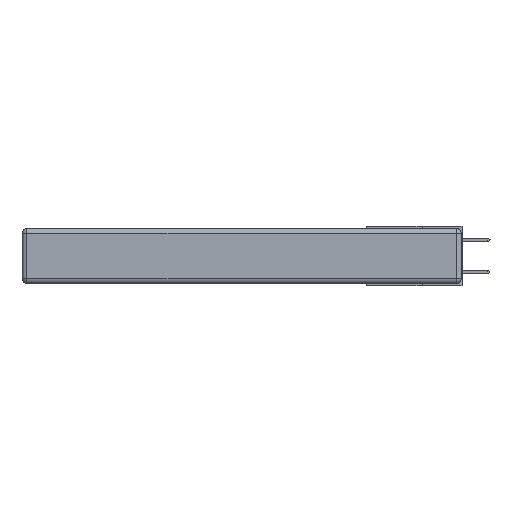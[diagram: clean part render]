
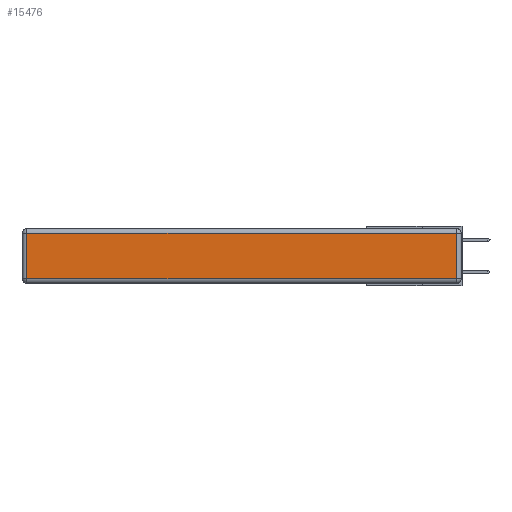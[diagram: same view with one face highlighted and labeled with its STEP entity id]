
A CAD part, left-side view. The second image highlights one B-rep face of the part: STEP entity #15476.
In plain terms, the highlighted planar face has unit normal (-1, 0, 0).
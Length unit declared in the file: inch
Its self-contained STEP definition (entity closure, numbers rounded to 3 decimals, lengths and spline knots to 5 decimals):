
#722 = CARTESIAN_POINT ( 'NONE',  ( 0., 0.03, -0.343 ) ) ;
#752 = VERTEX_POINT ( 'NONE', #2134 ) ;
#779 = CARTESIAN_POINT ( 'NONE',  ( 0., 0.03, -0.03 ) ) ;
#2084 = ORIENTED_EDGE ( 'NONE', *, *, #11543, .T. ) ;
#2134 = CARTESIAN_POINT ( 'NONE',  ( 0., 0.03, -0.313 ) ) ;
#2245 = PLANE ( 'NONE',  #8259 ) ;
#2355 = CARTESIAN_POINT ( 'NONE',  ( 0., 0., -0.343 ) ) ;
#2886 = LINE ( 'NONE', #722, #6823 ) ;
#3375 = VECTOR ( 'NONE', #6549, 39.37008 ) ;
#3705 = ORIENTED_EDGE ( 'NONE', *, *, #7056, .T. ) ;
#4206 = EDGE_CURVE ( 'NONE', #7280, #14655, #16331, .T. ) ;
#4642 = FACE_OUTER_BOUND ( 'NONE', #12273, .T. ) ;
#4744 = EDGE_CURVE ( 'NONE', #6863, #7280, #8169, .T. ) ;
#4990 = DIRECTION ( 'NONE',  ( 0., 0., 1. ) ) ;
#5026 = DIRECTION ( 'NONE',  ( 0., 1., 0. ) ) ;
#5149 = DIRECTION ( 'NONE',  ( 0., 0., 1. ) ) ;
#6549 = DIRECTION ( 'NONE',  ( 0., 0., -1. ) ) ;
#6823 = VECTOR ( 'NONE', #5149, 39.37008 ) ;
#6863 = VERTEX_POINT ( 'NONE', #779 ) ;
#7056 = EDGE_CURVE ( 'NONE', #14655, #752, #17276, .T. ) ;
#7280 = VERTEX_POINT ( 'NONE', #12853 ) ;
#7327 = DIRECTION ( 'NONE',  ( 0., -1., 0. ) ) ;
#7970 = CARTESIAN_POINT ( 'NONE',  ( 0., 2.72, -0.313 ) ) ;
#8169 = LINE ( 'NONE', #13023, #11747 ) ;
#8259 = AXIS2_PLACEMENT_3D ( 'NONE', #2355, #11708, #4990 ) ;
#10047 = ORIENTED_EDGE ( 'NONE', *, *, #4744, .T. ) ;
#11543 = EDGE_CURVE ( 'NONE', #752, #6863, #2886, .T. ) ;
#11708 = DIRECTION ( 'NONE',  ( -1., 0., 0. ) ) ;
#11747 = VECTOR ( 'NONE', #5026, 39.37008 ) ;
#12273 = EDGE_LOOP ( 'NONE', ( #3705, #2084, #10047, #16227 ) ) ;
#12853 = CARTESIAN_POINT ( 'NONE',  ( 0., 2.72, -0.03 ) ) ;
#13023 = CARTESIAN_POINT ( 'NONE',  ( 0., 2.75, -0.03 ) ) ;
#13732 = VECTOR ( 'NONE', #7327, 39.37008 ) ;
#14655 = VERTEX_POINT ( 'NONE', #7970 ) ;
#14743 = CARTESIAN_POINT ( 'NONE',  ( 0., 2.72, -0.343 ) ) ;
#15476 = ADVANCED_FACE ( 'NONE', ( #4642 ), #2245, .T. ) ;
#16227 = ORIENTED_EDGE ( 'NONE', *, *, #4206, .T. ) ;
#16331 = LINE ( 'NONE', #14743, #3375 ) ;
#16573 = CARTESIAN_POINT ( 'NONE',  ( 0., 0., -0.313 ) ) ;
#17276 = LINE ( 'NONE', #16573, #13732 ) ;
